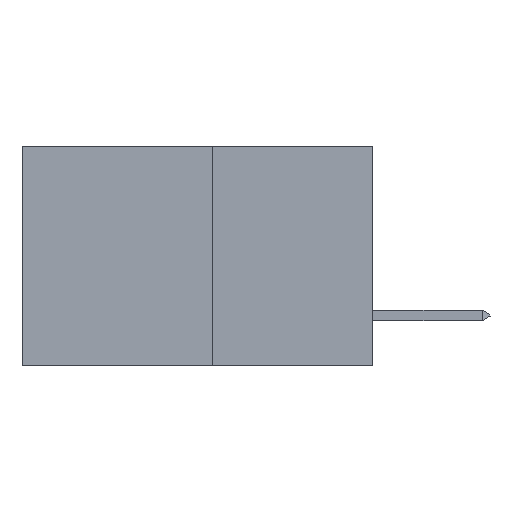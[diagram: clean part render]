
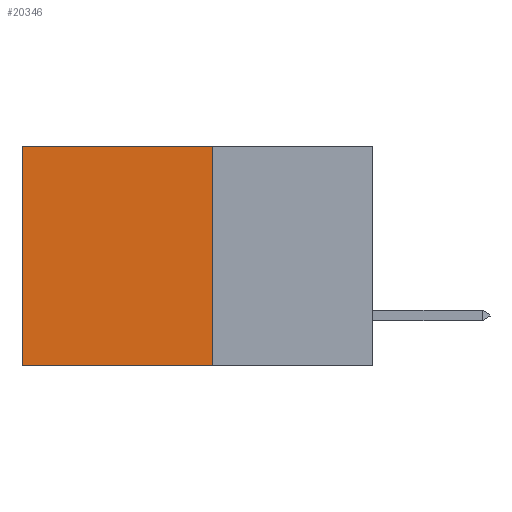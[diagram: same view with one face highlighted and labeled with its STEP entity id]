
A CAD part, left-side view. The second image highlights one B-rep face of the part: STEP entity #20346.
In plain terms, the highlighted planar face has unit normal (-1, 0, 0).
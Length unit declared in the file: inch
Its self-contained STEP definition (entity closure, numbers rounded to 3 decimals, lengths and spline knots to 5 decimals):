
#1981 = ORIENTED_EDGE ( 'NONE', *, *, #25741, .T. ) ;
#2818 = LINE ( 'NONE', #4717, #15594 ) ;
#3287 = PLANE ( 'NONE',  #6405 ) ;
#3567 = ORIENTED_EDGE ( 'NONE', *, *, #7410, .F. ) ;
#4717 = CARTESIAN_POINT ( 'NONE',  ( 0.277, 0.59, -0.37 ) ) ;
#5281 = VECTOR ( 'NONE', #22936, 39.37008 ) ;
#5309 = CARTESIAN_POINT ( 'NONE',  ( 0.277, 0.27, -0.37 ) ) ;
#6170 = ORIENTED_EDGE ( 'NONE', *, *, #21803, .F. ) ;
#6405 = AXIS2_PLACEMENT_3D ( 'NONE', #18519, #28506, #13574 ) ;
#6851 = CARTESIAN_POINT ( 'NONE',  ( 0.277, 0.27, -0.37 ) ) ;
#6898 = VECTOR ( 'NONE', #14419, 39.37008 ) ;
#7014 = CARTESIAN_POINT ( 'NONE',  ( 0.277, 0.27, -0.37 ) ) ;
#7104 = VECTOR ( 'NONE', #21596, 39.37008 ) ;
#7410 = EDGE_CURVE ( 'NONE', #30653, #16159, #20323, .T. ) ;
#9882 = DIRECTION ( 'NONE',  ( 0., 0., -1. ) ) ;
#11229 = CARTESIAN_POINT ( 'NONE',  ( 0.277, 0.27, 0. ) ) ;
#12135 = FACE_OUTER_BOUND ( 'NONE', #18703, .T. ) ;
#13574 = DIRECTION ( 'NONE',  ( 0., 0., -1. ) ) ;
#14419 = DIRECTION ( 'NONE',  ( 0., 1., 0. ) ) ;
#15177 = CARTESIAN_POINT ( 'NONE',  ( 0.277, 0.59, 0. ) ) ;
#15594 = VECTOR ( 'NONE', #9882, 39.37008 ) ;
#16159 = VERTEX_POINT ( 'NONE', #26723 ) ;
#18519 = CARTESIAN_POINT ( 'NONE',  ( 0.277, 0.27, -0.37 ) ) ;
#18703 = EDGE_LOOP ( 'NONE', ( #28254, #3567, #6170, #1981 ) ) ;
#18774 = LINE ( 'NONE', #5309, #5281 ) ;
#19115 = CARTESIAN_POINT ( 'NONE',  ( 0.277, 0.27, 0. ) ) ;
#20323 = LINE ( 'NONE', #6851, #6898 ) ;
#20346 = ADVANCED_FACE ( 'NONE', ( #12135 ), #3287, .F. ) ;
#20539 = LINE ( 'NONE', #19115, #7104 ) ;
#21085 = VERTEX_POINT ( 'NONE', #11229 ) ;
#21596 = DIRECTION ( 'NONE',  ( 0., 1., 0. ) ) ;
#21803 = EDGE_CURVE ( 'NONE', #21085, #30653, #18774, .T. ) ;
#22309 = EDGE_CURVE ( 'NONE', #30030, #16159, #2818, .T. ) ;
#22936 = DIRECTION ( 'NONE',  ( 0., 0., -1. ) ) ;
#25741 = EDGE_CURVE ( 'NONE', #21085, #30030, #20539, .T. ) ;
#26723 = CARTESIAN_POINT ( 'NONE',  ( 0.277, 0.59, -0.37 ) ) ;
#28254 = ORIENTED_EDGE ( 'NONE', *, *, #22309, .T. ) ;
#28506 = DIRECTION ( 'NONE',  ( 1., 0., 0. ) ) ;
#30030 = VERTEX_POINT ( 'NONE', #15177 ) ;
#30653 = VERTEX_POINT ( 'NONE', #7014 ) ;
